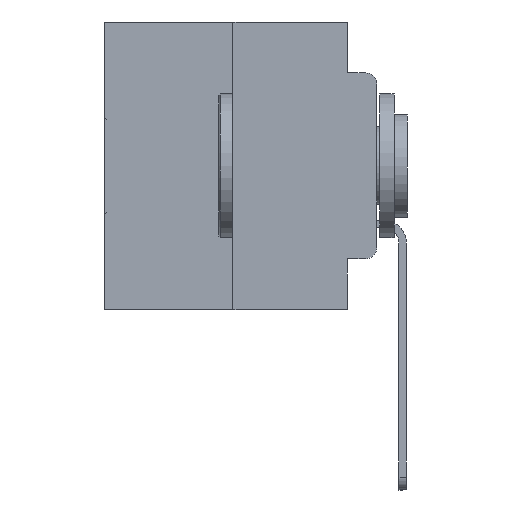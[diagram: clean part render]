
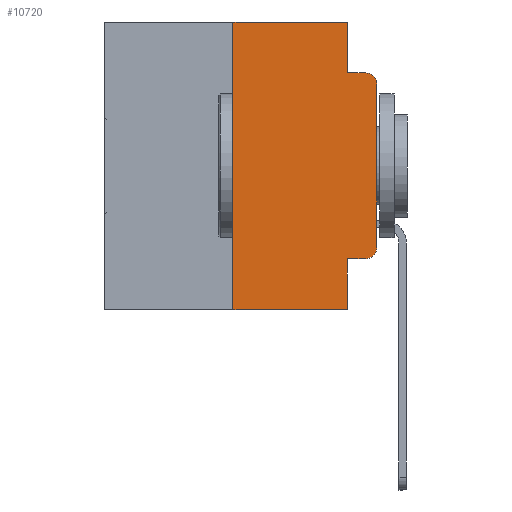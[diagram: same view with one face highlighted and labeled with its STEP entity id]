
A CAD part, left-side view. The second image highlights one B-rep face of the part: STEP entity #10720.
In plain terms, the highlighted planar face has unit normal (-1, 0, 0).
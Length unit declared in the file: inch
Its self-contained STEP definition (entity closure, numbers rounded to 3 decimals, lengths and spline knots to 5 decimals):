
#172 = FACE_OUTER_BOUND ( 'NONE', #27993, .T. ) ;
#364 = VERTEX_POINT ( 'NONE', #18066 ) ;
#535 = CARTESIAN_POINT ( 'NONE',  ( 0., 0.25, 0. ) ) ;
#1020 = DIRECTION ( 'NONE',  ( 0., 0., -1. ) ) ;
#1175 = EDGE_CURVE ( 'NONE', #5813, #364, #21095, .T. ) ;
#1446 = VERTEX_POINT ( 'NONE', #22972 ) ;
#1601 = CARTESIAN_POINT ( 'NONE',  ( 0., 0.051, 0. ) ) ;
#1766 = CARTESIAN_POINT ( 'NONE',  ( 0., 0.473, 0. ) ) ;
#1811 = ORIENTED_EDGE ( 'NONE', *, *, #19011, .F. ) ;
#2202 = CARTESIAN_POINT ( 'NONE',  ( 0., 0.02, -0.1085 ) ) ;
#2676 = VECTOR ( 'NONE', #19008, 39.37008 ) ;
#3126 = CARTESIAN_POINT ( 'NONE',  ( 0., 0.02, -0.3915 ) ) ;
#3587 = VERTEX_POINT ( 'NONE', #30027 ) ;
#4175 = DIRECTION ( 'NONE',  ( 0., 0., -1. ) ) ;
#4343 = DIRECTION ( 'NONE',  ( 0., 0., -1. ) ) ;
#4572 = ORIENTED_EDGE ( 'NONE', *, *, #1175, .F. ) ;
#4780 = DIRECTION ( 'NONE',  ( 0., 0., -1. ) ) ;
#5699 = DIRECTION ( 'NONE',  ( 0., 0., -1. ) ) ;
#5752 = EDGE_CURVE ( 'NONE', #7825, #364, #13344, .T. ) ;
#5803 = CARTESIAN_POINT ( 'NONE',  ( 0., 0.051, -0.4115 ) ) ;
#5813 = VERTEX_POINT ( 'NONE', #26644 ) ;
#6575 = ORIENTED_EDGE ( 'NONE', *, *, #8915, .F. ) ;
#7825 = VERTEX_POINT ( 'NONE', #18457 ) ;
#8325 = DIRECTION ( 'NONE',  ( 0., -1., 0. ) ) ;
#8915 = EDGE_CURVE ( 'NONE', #3587, #14620, #27991, .T. ) ;
#9065 = ORIENTED_EDGE ( 'NONE', *, *, #12664, .T. ) ;
#9068 = VECTOR ( 'NONE', #20178, 39.37008 ) ;
#9397 = LINE ( 'NONE', #16670, #2676 ) ;
#9614 = VERTEX_POINT ( 'NONE', #14469 ) ;
#9867 = CARTESIAN_POINT ( 'NONE',  ( 0., 0.051, -0.0885 ) ) ;
#10720 = ADVANCED_FACE ( 'NONE', ( #172 ), #16634, .F. ) ;
#11024 = CIRCLE ( 'NONE', #26827, 0.02 ) ;
#11112 = VECTOR ( 'NONE', #1020, 39.37008 ) ;
#11623 = EDGE_CURVE ( 'NONE', #16862, #13477, #27201, .T. ) ;
#11871 = LINE ( 'NONE', #22991, #11112 ) ;
#12059 = ORIENTED_EDGE ( 'NONE', *, *, #28000, .F. ) ;
#12664 = EDGE_CURVE ( 'NONE', #9614, #7825, #14733, .T. ) ;
#12862 = ORIENTED_EDGE ( 'NONE', *, *, #11623, .T. ) ;
#13123 = CARTESIAN_POINT ( 'NONE',  ( 0., 0., 0. ) ) ;
#13232 = VECTOR ( 'NONE', #15527, 39.37008 ) ;
#13344 = CIRCLE ( 'NONE', #21412, 0.02 ) ;
#13378 = LINE ( 'NONE', #1601, #31168 ) ;
#13477 = VERTEX_POINT ( 'NONE', #25824 ) ;
#14137 = VECTOR ( 'NONE', #24161, 39.37008 ) ;
#14469 = CARTESIAN_POINT ( 'NONE',  ( 0., 0., -0.3915 ) ) ;
#14620 = VERTEX_POINT ( 'NONE', #535 ) ;
#14733 = LINE ( 'NONE', #13123, #13232 ) ;
#15094 = CARTESIAN_POINT ( 'NONE',  ( 0., 0.051, 0. ) ) ;
#15454 = CARTESIAN_POINT ( 'NONE',  ( 0., 0.25, 0. ) ) ;
#15527 = DIRECTION ( 'NONE',  ( 0., 0., 1. ) ) ;
#16634 = PLANE ( 'NONE',  #25285 ) ;
#16670 = CARTESIAN_POINT ( 'NONE',  ( 0., 0.473, 0. ) ) ;
#16862 = VERTEX_POINT ( 'NONE', #27523 ) ;
#17055 = EDGE_CURVE ( 'NONE', #19930, #5813, #13378, .T. ) ;
#18007 = ORIENTED_EDGE ( 'NONE', *, *, #17055, .F. ) ;
#18048 = EDGE_CURVE ( 'NONE', #13477, #9614, #11024, .T. ) ;
#18066 = CARTESIAN_POINT ( 'NONE',  ( 0., 0.02, -0.0885 ) ) ;
#18457 = CARTESIAN_POINT ( 'NONE',  ( 0., 0., -0.1085 ) ) ;
#18972 = DIRECTION ( 'NONE',  ( 1., 0., 0. ) ) ;
#19008 = DIRECTION ( 'NONE',  ( 0., -1., 0. ) ) ;
#19011 = EDGE_CURVE ( 'NONE', #14620, #19930, #9397, .T. ) ;
#19373 = DIRECTION ( 'NONE',  ( -1., 0., 0. ) ) ;
#19532 = ORIENTED_EDGE ( 'NONE', *, *, #18048, .T. ) ;
#19930 = VERTEX_POINT ( 'NONE', #15094 ) ;
#20178 = DIRECTION ( 'NONE',  ( 0., 0., 1. ) ) ;
#20240 = DIRECTION ( 'NONE',  ( -1., 0., 0. ) ) ;
#20252 = ORIENTED_EDGE ( 'NONE', *, *, #29009, .T. ) ;
#20975 = VECTOR ( 'NONE', #8325, 39.37008 ) ;
#21095 = LINE ( 'NONE', #9867, #14137 ) ;
#21412 = AXIS2_PLACEMENT_3D ( 'NONE', #2202, #19373, #4780 ) ;
#22972 = CARTESIAN_POINT ( 'NONE',  ( 0., 0.051, -0.5 ) ) ;
#22991 = CARTESIAN_POINT ( 'NONE',  ( 0., 0.051, 0. ) ) ;
#24161 = DIRECTION ( 'NONE',  ( 0., -1., 0. ) ) ;
#24218 = CARTESIAN_POINT ( 'NONE',  ( 0., 0.473, -0.5 ) ) ;
#25285 = AXIS2_PLACEMENT_3D ( 'NONE', #1766, #18972, #4343 ) ;
#25824 = CARTESIAN_POINT ( 'NONE',  ( 0., 0.02, -0.4115 ) ) ;
#26564 = DIRECTION ( 'NONE',  ( 0., -1., 0. ) ) ;
#26644 = CARTESIAN_POINT ( 'NONE',  ( 0., 0.051, -0.0885 ) ) ;
#26827 = AXIS2_PLACEMENT_3D ( 'NONE', #3126, #20240, #5699 ) ;
#27201 = LINE ( 'NONE', #5803, #20975 ) ;
#27523 = CARTESIAN_POINT ( 'NONE',  ( 0., 0.051, -0.4115 ) ) ;
#27991 = LINE ( 'NONE', #15454, #9068 ) ;
#27993 = EDGE_LOOP ( 'NONE', ( #9065, #30969, #4572, #18007, #1811, #6575, #20252, #12059, #12862, #19532 ) ) ;
#28000 = EDGE_CURVE ( 'NONE', #16862, #1446, #11871, .T. ) ;
#29009 = EDGE_CURVE ( 'NONE', #3587, #1446, #31169, .T. ) ;
#30027 = CARTESIAN_POINT ( 'NONE',  ( 0., 0.25, -0.5 ) ) ;
#30479 = VECTOR ( 'NONE', #26564, 39.37008 ) ;
#30969 = ORIENTED_EDGE ( 'NONE', *, *, #5752, .T. ) ;
#31168 = VECTOR ( 'NONE', #4175, 39.37008 ) ;
#31169 = LINE ( 'NONE', #24218, #30479 ) ;
